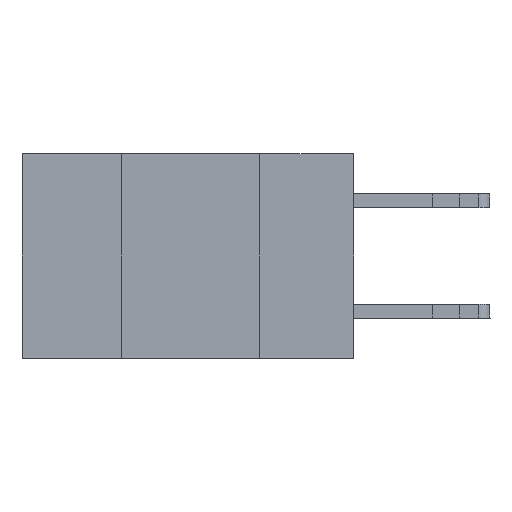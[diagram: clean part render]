
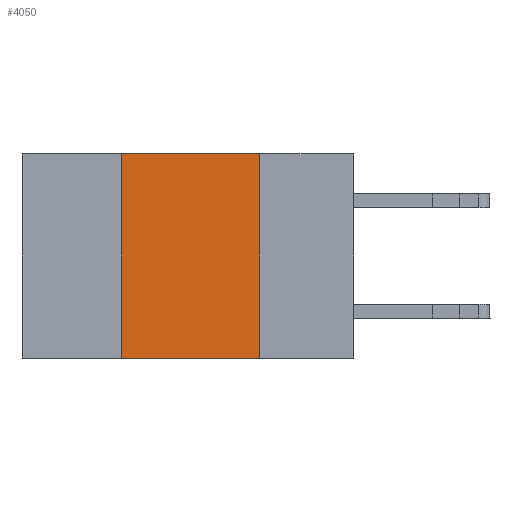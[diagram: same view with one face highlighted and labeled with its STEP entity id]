
A CAD part, left-side view. The second image highlights one B-rep face of the part: STEP entity #4050.
In plain terms, the highlighted planar face has unit normal (-1, 0, 0).
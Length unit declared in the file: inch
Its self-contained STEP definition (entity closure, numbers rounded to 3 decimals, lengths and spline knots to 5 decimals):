
#164 = ORIENTED_EDGE ( 'NONE', *, *, #18488, .F. ) ;
#549 = EDGE_CURVE ( 'NONE', #1479, #3837, #6223, .T. ) ;
#1479 = VERTEX_POINT ( 'NONE', #10179 ) ;
#1619 = DIRECTION ( 'NONE',  ( 0., -1., 0. ) ) ;
#1992 = VECTOR ( 'NONE', #1619, 39.37008 ) ;
#2533 = VECTOR ( 'NONE', #18324, 39.37008 ) ;
#3837 = VERTEX_POINT ( 'NONE', #20440 ) ;
#3884 = DIRECTION ( 'NONE',  ( 1., 0., 0. ) ) ;
#4050 = ADVANCED_FACE ( 'NONE', ( #5570 ), #14052, .F. ) ;
#4291 = VERTEX_POINT ( 'NONE', #6309 ) ;
#5570 = FACE_OUTER_BOUND ( 'NONE', #13344, .T. ) ;
#6223 = LINE ( 'NONE', #8149, #10199 ) ;
#6309 = CARTESIAN_POINT ( 'NONE',  ( 0., 0.17, -0.37 ) ) ;
#8149 = CARTESIAN_POINT ( 'NONE',  ( 0., 0.6, 0. ) ) ;
#8586 = CARTESIAN_POINT ( 'NONE',  ( 0., 0.6, -0.37 ) ) ;
#8930 = CARTESIAN_POINT ( 'NONE',  ( 0., 0.42, -0.37 ) ) ;
#9811 = LINE ( 'NONE', #17092, #18372 ) ;
#10179 = CARTESIAN_POINT ( 'NONE',  ( 0., 0.42, 0. ) ) ;
#10199 = VECTOR ( 'NONE', #21222, 39.37008 ) ;
#10943 = EDGE_CURVE ( 'NONE', #19226, #4291, #15097, .T. ) ;
#11297 = EDGE_CURVE ( 'NONE', #19226, #1479, #16172, .T. ) ;
#12884 = ORIENTED_EDGE ( 'NONE', *, *, #549, .F. ) ;
#13344 = EDGE_LOOP ( 'NONE', ( #164, #12884, #17056, #16683 ) ) ;
#14052 = PLANE ( 'NONE',  #19602 ) ;
#15097 = LINE ( 'NONE', #8586, #1992 ) ;
#15303 = DIRECTION ( 'NONE',  ( 0., 0., -1. ) ) ;
#15797 = DIRECTION ( 'NONE',  ( 0., 0., -1. ) ) ;
#16172 = LINE ( 'NONE', #18395, #2533 ) ;
#16683 = ORIENTED_EDGE ( 'NONE', *, *, #10943, .T. ) ;
#17056 = ORIENTED_EDGE ( 'NONE', *, *, #11297, .F. ) ;
#17092 = CARTESIAN_POINT ( 'NONE',  ( 0., 0.17, 0. ) ) ;
#18324 = DIRECTION ( 'NONE',  ( 0., 0., 1. ) ) ;
#18372 = VECTOR ( 'NONE', #15303, 39.37008 ) ;
#18395 = CARTESIAN_POINT ( 'NONE',  ( 0., 0.42, 0. ) ) ;
#18488 = EDGE_CURVE ( 'NONE', #3837, #4291, #9811, .T. ) ;
#19226 = VERTEX_POINT ( 'NONE', #8930 ) ;
#19263 = CARTESIAN_POINT ( 'NONE',  ( 0., 0.6, 0. ) ) ;
#19602 = AXIS2_PLACEMENT_3D ( 'NONE', #19263, #3884, #15797 ) ;
#20440 = CARTESIAN_POINT ( 'NONE',  ( 0., 0.17, 0. ) ) ;
#21222 = DIRECTION ( 'NONE',  ( 0., -1., 0. ) ) ;
